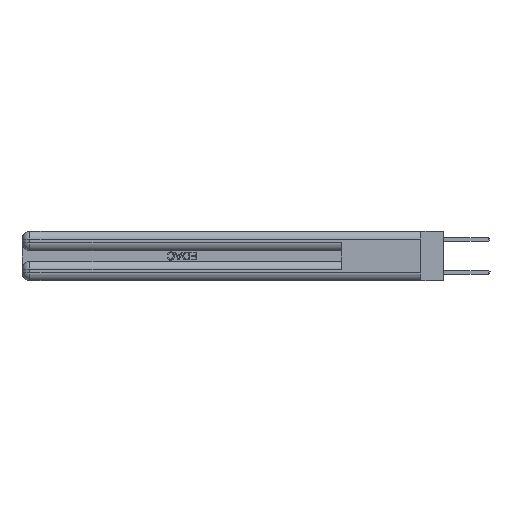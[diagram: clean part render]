
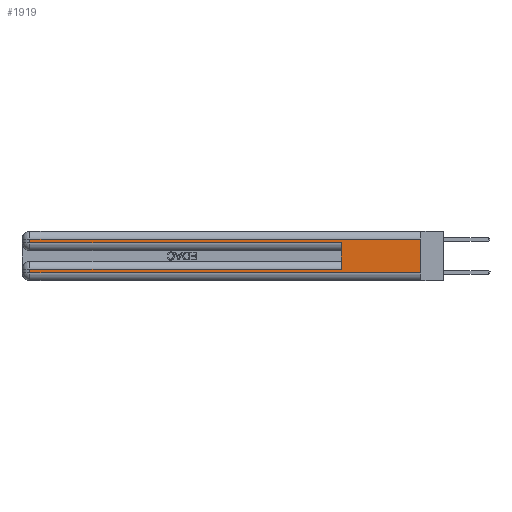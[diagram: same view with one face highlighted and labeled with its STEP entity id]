
A CAD part, left-side view. The second image highlights one B-rep face of the part: STEP entity #1919.
In plain terms, the highlighted planar face has unit normal (-1, 0, 0).
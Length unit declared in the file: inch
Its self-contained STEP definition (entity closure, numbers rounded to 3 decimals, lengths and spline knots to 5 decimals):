
#172 = ORIENTED_EDGE ( 'NONE', *, *, #36900, .F. ) ;
#294 = VERTEX_POINT ( 'NONE', #8883 ) ;
#528 = ORIENTED_EDGE ( 'NONE', *, *, #35612, .F. ) ;
#566 = FACE_OUTER_BOUND ( 'NONE', #12844, .T. ) ;
#1120 = LINE ( 'NONE', #12637, #19322 ) ;
#1919 = ADVANCED_FACE ( 'NONE', ( #566 ), #3400, .F. ) ;
#2650 = LINE ( 'NONE', #33676, #26616 ) ;
#3027 = CARTESIAN_POINT ( 'NONE',  ( 0., 0., 0.37 ) ) ;
#3400 = PLANE ( 'NONE',  #5703 ) ;
#3440 = CARTESIAN_POINT ( 'NONE',  ( 0., 2.94, 0.06 ) ) ;
#3755 = DIRECTION ( 'NONE',  ( 0., 0., -1. ) ) ;
#4374 = DIRECTION ( 'NONE',  ( 0., 0., 1. ) ) ;
#5147 = DIRECTION ( 'NONE',  ( 0., 1., 0. ) ) ;
#5152 = VECTOR ( 'NONE', #4374, 39.37008 ) ;
#5703 = AXIS2_PLACEMENT_3D ( 'NONE', #12082, #23637, #35171 ) ;
#8049 = LINE ( 'NONE', #19571, #18089 ) ;
#8883 = CARTESIAN_POINT ( 'NONE',  ( 0., 0.6, 0.285 ) ) ;
#8985 = VERTEX_POINT ( 'NONE', #27884 ) ;
#9409 = EDGE_CURVE ( 'NONE', #26731, #13442, #31135, .T. ) ;
#9798 = DIRECTION ( 'NONE',  ( 0., 0., -1. ) ) ;
#10562 = VECTOR ( 'NONE', #34524, 39.37008 ) ;
#10577 = CARTESIAN_POINT ( 'NONE',  ( 0., 0., 0.31 ) ) ;
#10772 = CARTESIAN_POINT ( 'NONE',  ( 0., 0.6, 0.085 ) ) ;
#11271 = VERTEX_POINT ( 'NONE', #32401 ) ;
#11439 = CARTESIAN_POINT ( 'NONE',  ( 0., 0., 0.06 ) ) ;
#11477 = LINE ( 'NONE', #19973, #12198 ) ;
#12082 = CARTESIAN_POINT ( 'NONE',  ( 0., 0., 0.37 ) ) ;
#12198 = VECTOR ( 'NONE', #37206, 39.37008 ) ;
#12637 = CARTESIAN_POINT ( 'NONE',  ( 0., 2.94, 0.37 ) ) ;
#12844 = EDGE_LOOP ( 'NONE', ( #528, #26991, #17917, #26870, #172, #28853, #31389, #25504 ) ) ;
#13442 = VERTEX_POINT ( 'NONE', #28532 ) ;
#13789 = LINE ( 'NONE', #18732, #5152 ) ;
#14863 = VERTEX_POINT ( 'NONE', #10577 ) ;
#17437 = EDGE_CURVE ( 'NONE', #32198, #11271, #2650, .T. ) ;
#17606 = CARTESIAN_POINT ( 'NONE',  ( 0., 2.94, 0.31 ) ) ;
#17714 = EDGE_CURVE ( 'NONE', #8985, #26731, #1120, .T. ) ;
#17917 = ORIENTED_EDGE ( 'NONE', *, *, #17437, .T. ) ;
#18089 = VECTOR ( 'NONE', #22243, 39.37008 ) ;
#18732 = CARTESIAN_POINT ( 'NONE',  ( 0., 0.6, 0.145 ) ) ;
#19322 = VECTOR ( 'NONE', #9798, 39.37008 ) ;
#19571 = CARTESIAN_POINT ( 'NONE',  ( 0., 0., 0.285 ) ) ;
#19973 = CARTESIAN_POINT ( 'NONE',  ( 0., 0., 0.31 ) ) ;
#22243 = DIRECTION ( 'NONE',  ( 0., -1., 0. ) ) ;
#23637 = DIRECTION ( 'NONE',  ( 1., 0., 0. ) ) ;
#24119 = EDGE_CURVE ( 'NONE', #11271, #294, #8049, .T. ) ;
#25023 = CARTESIAN_POINT ( 'NONE',  ( 0., 0., 0.085 ) ) ;
#25504 = ORIENTED_EDGE ( 'NONE', *, *, #9409, .T. ) ;
#26616 = VECTOR ( 'NONE', #30854, 39.37008 ) ;
#26731 = VERTEX_POINT ( 'NONE', #3440 ) ;
#26870 = ORIENTED_EDGE ( 'NONE', *, *, #24119, .T. ) ;
#26991 = ORIENTED_EDGE ( 'NONE', *, *, #28904, .T. ) ;
#27884 = CARTESIAN_POINT ( 'NONE',  ( 0., 2.94, 0.085 ) ) ;
#28532 = CARTESIAN_POINT ( 'NONE',  ( 0., 0., 0.06 ) ) ;
#28853 = ORIENTED_EDGE ( 'NONE', *, *, #33289, .T. ) ;
#28904 = EDGE_CURVE ( 'NONE', #14863, #32198, #11477, .T. ) ;
#29678 = LINE ( 'NONE', #3027, #31093 ) ;
#30854 = DIRECTION ( 'NONE',  ( 0., 0., -1. ) ) ;
#31093 = VECTOR ( 'NONE', #3755, 39.37008 ) ;
#31135 = LINE ( 'NONE', #11439, #10562 ) ;
#31389 = ORIENTED_EDGE ( 'NONE', *, *, #17714, .T. ) ;
#32198 = VERTEX_POINT ( 'NONE', #17606 ) ;
#32367 = VECTOR ( 'NONE', #5147, 39.37008 ) ;
#32401 = CARTESIAN_POINT ( 'NONE',  ( 0., 2.94, 0.285 ) ) ;
#33289 = EDGE_CURVE ( 'NONE', #36927, #8985, #33912, .T. ) ;
#33676 = CARTESIAN_POINT ( 'NONE',  ( 0., 2.94, 0.37 ) ) ;
#33912 = LINE ( 'NONE', #25023, #32367 ) ;
#34524 = DIRECTION ( 'NONE',  ( 0., -1., 0. ) ) ;
#35171 = DIRECTION ( 'NONE',  ( 0., 0., -1. ) ) ;
#35612 = EDGE_CURVE ( 'NONE', #14863, #13442, #29678, .T. ) ;
#36900 = EDGE_CURVE ( 'NONE', #36927, #294, #13789, .T. ) ;
#36927 = VERTEX_POINT ( 'NONE', #10772 ) ;
#37206 = DIRECTION ( 'NONE',  ( 0., 1., 0. ) ) ;
